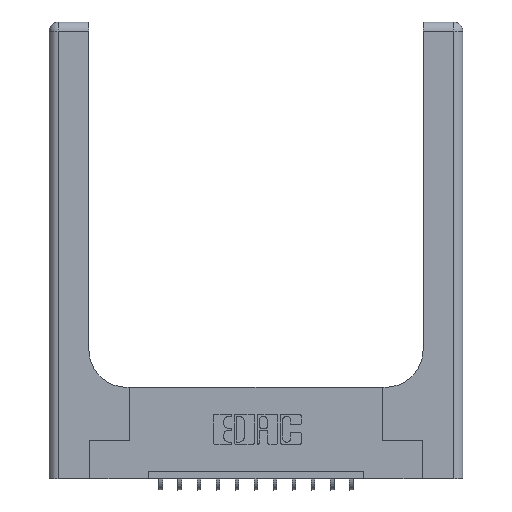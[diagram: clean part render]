
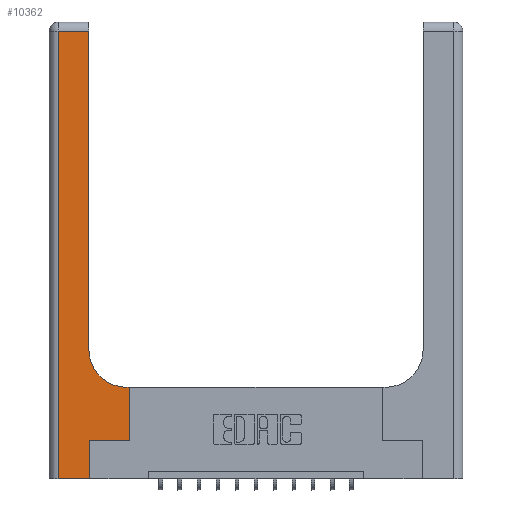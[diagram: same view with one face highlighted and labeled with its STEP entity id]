
A CAD part, top view. The second image highlights one B-rep face of the part: STEP entity #10362.
In plain terms, the highlighted planar face has unit normal (0, 0, 1).
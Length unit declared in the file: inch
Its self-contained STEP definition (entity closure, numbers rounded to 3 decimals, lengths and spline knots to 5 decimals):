
#14 = CARTESIAN_POINT ( 'NONE',  ( 0.528, 0.25, 0.37 ) ) ;
#419 = ORIENTED_EDGE ( 'NONE', *, *, #16292, .T. ) ;
#456 = EDGE_CURVE ( 'NONE', #10065, #4638, #10198, .T. ) ;
#1182 = FACE_OUTER_BOUND ( 'NONE', #2008, .T. ) ;
#1614 = LINE ( 'NONE', #13165, #15739 ) ;
#2008 = EDGE_LOOP ( 'NONE', ( #10186, #2189, #8983, #419, #16533, #6896, #4449, #9797, #2963 ) ) ;
#2189 = ORIENTED_EDGE ( 'NONE', *, *, #15813, .T. ) ;
#2848 = EDGE_CURVE ( 'NONE', #5954, #10065, #1614, .T. ) ;
#2963 = ORIENTED_EDGE ( 'NONE', *, *, #7440, .T. ) ;
#3734 = VECTOR ( 'NONE', #5036, 39.37008 ) ;
#3997 = LINE ( 'NONE', #6285, #4360 ) ;
#4070 = DIRECTION ( 'NONE',  ( 0., 1., 0. ) ) ;
#4360 = VECTOR ( 'NONE', #4070, 39.37008 ) ;
#4376 = LINE ( 'NONE', #14848, #10217 ) ;
#4449 = ORIENTED_EDGE ( 'NONE', *, *, #456, .T. ) ;
#4638 = VERTEX_POINT ( 'NONE', #14224 ) ;
#4831 = VERTEX_POINT ( 'NONE', #12846 ) ;
#5036 = DIRECTION ( 'NONE',  ( -1., 0., 0. ) ) ;
#5261 = CARTESIAN_POINT ( 'NONE',  ( 0.26, 0.85, 0.37 ) ) ;
#5900 = DIRECTION ( 'NONE',  ( 1., 0., 0. ) ) ;
#5954 = VERTEX_POINT ( 'NONE', #9209 ) ;
#5972 = VERTEX_POINT ( 'NONE', #6600 ) ;
#6081 = CARTESIAN_POINT ( 'NONE',  ( 0., 3., 0.37 ) ) ;
#6238 = LINE ( 'NONE', #12479, #8065 ) ;
#6285 = CARTESIAN_POINT ( 'NONE',  ( 0.26, 3., 0.37 ) ) ;
#6322 = DIRECTION ( 'NONE',  ( 0., 0., -1. ) ) ;
#6600 = CARTESIAN_POINT ( 'NONE',  ( 0.51, 0.6, 0.37 ) ) ;
#6896 = ORIENTED_EDGE ( 'NONE', *, *, #2848, .T. ) ;
#7314 = AXIS2_PLACEMENT_3D ( 'NONE', #6081, #6322, #8890 ) ;
#7440 = EDGE_CURVE ( 'NONE', #5972, #7541, #10196, .T. ) ;
#7541 = VERTEX_POINT ( 'NONE', #5261 ) ;
#7714 = DIRECTION ( 'NONE',  ( 1., 0., 0. ) ) ;
#8060 = VECTOR ( 'NONE', #10707, 39.37008 ) ;
#8065 = VECTOR ( 'NONE', #5900, 39.37008 ) ;
#8078 = CARTESIAN_POINT ( 'NONE',  ( 0., 2.94, 0.37 ) ) ;
#8159 = EDGE_CURVE ( 'NONE', #15965, #5954, #9793, .T. ) ;
#8677 = CARTESIAN_POINT ( 'NONE',  ( 0.265, 0., 0.37 ) ) ;
#8822 = EDGE_CURVE ( 'NONE', #4831, #15032, #4376, .T. ) ;
#8890 = DIRECTION ( 'NONE',  ( -1., 0., 0. ) ) ;
#8983 = ORIENTED_EDGE ( 'NONE', *, *, #8822, .T. ) ;
#9209 = CARTESIAN_POINT ( 'NONE',  ( 0.265, 0.25, 0.37 ) ) ;
#9361 = LINE ( 'NONE', #8078, #8060 ) ;
#9655 = VECTOR ( 'NONE', #12191, 39.37008 ) ;
#9793 = LINE ( 'NONE', #16014, #9655 ) ;
#9797 = ORIENTED_EDGE ( 'NONE', *, *, #13696, .T. ) ;
#9846 = VECTOR ( 'NONE', #15394, 39.37008 ) ;
#10065 = VERTEX_POINT ( 'NONE', #14 ) ;
#10151 = CARTESIAN_POINT ( 'NONE',  ( 0.26, 0.6, 0.37 ) ) ;
#10186 = ORIENTED_EDGE ( 'NONE', *, *, #11403, .T. ) ;
#10196 = CIRCLE ( 'NONE', #14772, 0.25 ) ;
#10198 = LINE ( 'NONE', #11738, #9846 ) ;
#10217 = VECTOR ( 'NONE', #14589, 39.37008 ) ;
#10230 = LINE ( 'NONE', #10151, #3734 ) ;
#10362 = ADVANCED_FACE ( 'NONE', ( #1182 ), #16558, .F. ) ;
#10436 = DIRECTION ( 'NONE',  ( 0., 0., -1. ) ) ;
#10602 = DIRECTION ( 'NONE',  ( 1., 0., 0. ) ) ;
#10707 = DIRECTION ( 'NONE',  ( -1., 0., 0. ) ) ;
#11403 = EDGE_CURVE ( 'NONE', #7541, #13145, #3997, .T. ) ;
#11738 = CARTESIAN_POINT ( 'NONE',  ( 0.528, 0.25, 0.37 ) ) ;
#12191 = DIRECTION ( 'NONE',  ( 0., 1., 0. ) ) ;
#12479 = CARTESIAN_POINT ( 'NONE',  ( 0., 0., 0.37 ) ) ;
#12846 = CARTESIAN_POINT ( 'NONE',  ( 0.06, 2.94, 0.37 ) ) ;
#13120 = CARTESIAN_POINT ( 'NONE',  ( 0.06, 0., 0.37 ) ) ;
#13145 = VERTEX_POINT ( 'NONE', #16250 ) ;
#13165 = CARTESIAN_POINT ( 'NONE',  ( 0.265, 0.25, 0.37 ) ) ;
#13696 = EDGE_CURVE ( 'NONE', #4638, #5972, #10230, .T. ) ;
#14224 = CARTESIAN_POINT ( 'NONE',  ( 0.528, 0.6, 0.37 ) ) ;
#14589 = DIRECTION ( 'NONE',  ( 0., -1., 0. ) ) ;
#14772 = AXIS2_PLACEMENT_3D ( 'NONE', #15725, #10436, #7714 ) ;
#14848 = CARTESIAN_POINT ( 'NONE',  ( 0.06, 3., 0.37 ) ) ;
#15032 = VERTEX_POINT ( 'NONE', #13120 ) ;
#15394 = DIRECTION ( 'NONE',  ( 0., 1., 0. ) ) ;
#15725 = CARTESIAN_POINT ( 'NONE',  ( 0.51, 0.85, 0.37 ) ) ;
#15739 = VECTOR ( 'NONE', #10602, 39.37008 ) ;
#15813 = EDGE_CURVE ( 'NONE', #13145, #4831, #9361, .T. ) ;
#15965 = VERTEX_POINT ( 'NONE', #8677 ) ;
#16014 = CARTESIAN_POINT ( 'NONE',  ( 0.265, 0., 0.37 ) ) ;
#16250 = CARTESIAN_POINT ( 'NONE',  ( 0.26, 2.94, 0.37 ) ) ;
#16292 = EDGE_CURVE ( 'NONE', #15032, #15965, #6238, .T. ) ;
#16533 = ORIENTED_EDGE ( 'NONE', *, *, #8159, .T. ) ;
#16558 = PLANE ( 'NONE',  #7314 ) ;
